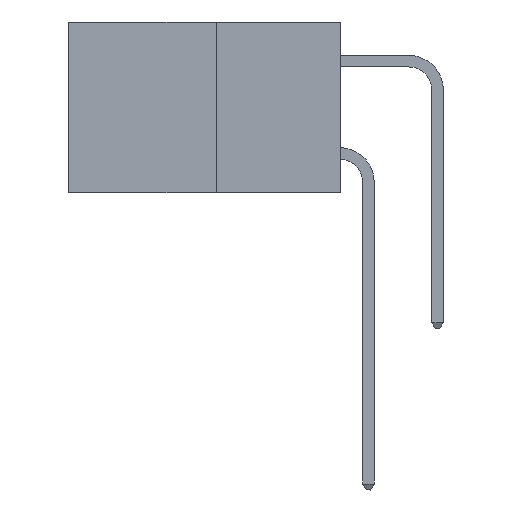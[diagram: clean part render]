
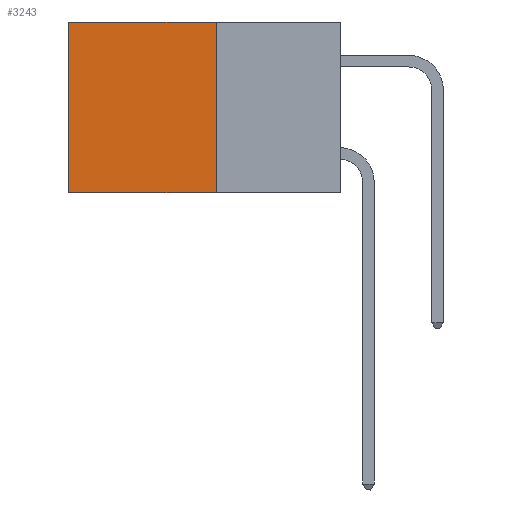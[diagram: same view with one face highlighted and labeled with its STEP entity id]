
A CAD part, left-side view. The second image highlights one B-rep face of the part: STEP entity #3243.
In plain terms, the highlighted planar face has unit normal (-1, 0, 0).
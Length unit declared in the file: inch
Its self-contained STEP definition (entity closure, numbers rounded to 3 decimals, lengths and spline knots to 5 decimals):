
#1146 = CARTESIAN_POINT ( 'NONE',  ( 0.277, 0.27, -0.37 ) ) ;
#1351 = EDGE_CURVE ( 'NONE', #7838, #4375, #2581, .T. ) ;
#1577 = CARTESIAN_POINT ( 'NONE',  ( 0.277, 0.59, -0.37 ) ) ;
#2085 = ORIENTED_EDGE ( 'NONE', *, *, #11858, .T. ) ;
#2211 = VECTOR ( 'NONE', #8376, 39.37008 ) ;
#2533 = ORIENTED_EDGE ( 'NONE', *, *, #12215, .F. ) ;
#2540 = DIRECTION ( 'NONE',  ( 0., 0., -1. ) ) ;
#2574 = PLANE ( 'NONE',  #7111 ) ;
#2581 = LINE ( 'NONE', #1577, #2211 ) ;
#2617 = CARTESIAN_POINT ( 'NONE',  ( 0.277, 0.59, 0. ) ) ;
#2629 = CARTESIAN_POINT ( 'NONE',  ( 0.277, 0.27, -0.37 ) ) ;
#2720 = DIRECTION ( 'NONE',  ( 1., 0., 0. ) ) ;
#3243 = ADVANCED_FACE ( 'NONE', ( #10554 ), #2574, .F. ) ;
#3521 = CARTESIAN_POINT ( 'NONE',  ( 0.277, 0.27, -0.37 ) ) ;
#4375 = VERTEX_POINT ( 'NONE', #5222 ) ;
#4668 = VERTEX_POINT ( 'NONE', #13480 ) ;
#5222 = CARTESIAN_POINT ( 'NONE',  ( 0.277, 0.59, -0.37 ) ) ;
#5465 = CARTESIAN_POINT ( 'NONE',  ( 0.277, 0.27, -0.37 ) ) ;
#7111 = AXIS2_PLACEMENT_3D ( 'NONE', #2629, #2720, #2540 ) ;
#7389 = DIRECTION ( 'NONE',  ( 0., 1., 0. ) ) ;
#7755 = DIRECTION ( 'NONE',  ( 0., 0., -1. ) ) ;
#7838 = VERTEX_POINT ( 'NONE', #2617 ) ;
#8311 = LINE ( 'NONE', #3521, #10661 ) ;
#8376 = DIRECTION ( 'NONE',  ( 0., 0., -1. ) ) ;
#8794 = VECTOR ( 'NONE', #7389, 39.37008 ) ;
#8812 = DIRECTION ( 'NONE',  ( 0., 1., 0. ) ) ;
#10103 = ORIENTED_EDGE ( 'NONE', *, *, #1351, .T. ) ;
#10554 = FACE_OUTER_BOUND ( 'NONE', #13772, .T. ) ;
#10661 = VECTOR ( 'NONE', #7755, 39.37008 ) ;
#11743 = LINE ( 'NONE', #12339, #8794 ) ;
#11858 = EDGE_CURVE ( 'NONE', #4668, #7838, #11743, .T. ) ;
#12037 = VERTEX_POINT ( 'NONE', #5465 ) ;
#12215 = EDGE_CURVE ( 'NONE', #4668, #12037, #8311, .T. ) ;
#12239 = EDGE_CURVE ( 'NONE', #12037, #4375, #13241, .T. ) ;
#12339 = CARTESIAN_POINT ( 'NONE',  ( 0.277, 0.27, 0. ) ) ;
#12940 = VECTOR ( 'NONE', #8812, 39.37008 ) ;
#13241 = LINE ( 'NONE', #1146, #12940 ) ;
#13480 = CARTESIAN_POINT ( 'NONE',  ( 0.277, 0.27, 0. ) ) ;
#13563 = ORIENTED_EDGE ( 'NONE', *, *, #12239, .F. ) ;
#13772 = EDGE_LOOP ( 'NONE', ( #10103, #13563, #2533, #2085 ) ) ;
